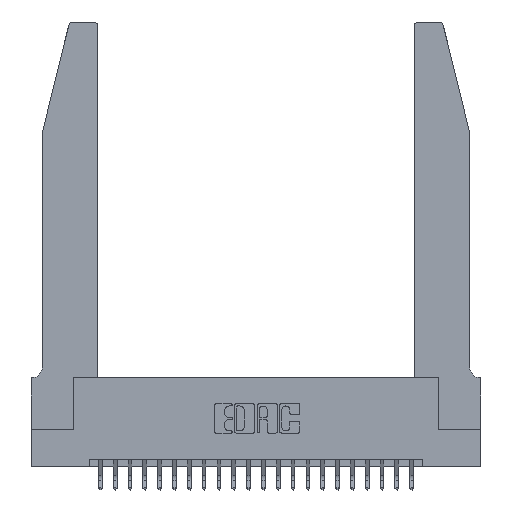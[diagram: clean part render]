
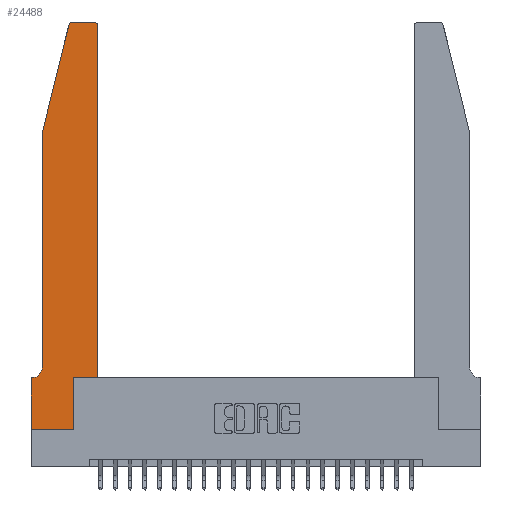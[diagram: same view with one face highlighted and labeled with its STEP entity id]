
A CAD part, top view. The second image highlights one B-rep face of the part: STEP entity #24488.
In plain terms, the highlighted planar face has unit normal (0, 0, 1).
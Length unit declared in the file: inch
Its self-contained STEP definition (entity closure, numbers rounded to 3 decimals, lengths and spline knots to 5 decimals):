
#172 = VERTEX_POINT ( 'NONE', #23364 ) ;
#546 = CARTESIAN_POINT ( 'NONE',  ( 0.2605, 2.75, 0.37 ) ) ;
#727 = CIRCLE ( 'NONE', #18479, 0.07 ) ;
#772 = CARTESIAN_POINT ( 'NONE',  ( 0.0055, 0.42, 0.37 ) ) ;
#1529 = CARTESIAN_POINT ( 'NONE',  ( 0., 0.35, 0.37 ) ) ;
#1618 = VERTEX_POINT ( 'NONE', #3143 ) ;
#1626 = EDGE_CURVE ( 'NONE', #13766, #11503, #6456, .T. ) ;
#1854 = VECTOR ( 'NONE', #22477, 39.37008 ) ;
#2359 = LINE ( 'NONE', #3358, #7561 ) ;
#2394 = EDGE_CURVE ( 'NONE', #13511, #3451, #6112, .T. ) ;
#2552 = DIRECTION ( 'NONE',  ( 0., -1., 0. ) ) ;
#2730 = VECTOR ( 'NONE', #21021, 39.37008 ) ;
#2745 = DIRECTION ( 'NONE',  ( 0., 0., 1. ) ) ;
#2781 = DIRECTION ( 'NONE',  ( -1., 0., 0. ) ) ;
#2784 = CARTESIAN_POINT ( 'NONE',  ( 0.284, 2.75, 0.37 ) ) ;
#2868 = DIRECTION ( 'NONE',  ( 0., 0., 1. ) ) ;
#2999 = VECTOR ( 'NONE', #14228, 39.37008 ) ;
#3043 = CARTESIAN_POINT ( 'NONE',  ( 0.4205, 2.72, 0.37 ) ) ;
#3143 = CARTESIAN_POINT ( 'NONE',  ( 0.0055, 0.35, 0.37 ) ) ;
#3145 = CARTESIAN_POINT ( 'NONE',  ( 0.0755, 2., 0.37 ) ) ;
#3358 = CARTESIAN_POINT ( 'NONE',  ( 0.2865, 0.35, 0.37 ) ) ;
#3451 = VERTEX_POINT ( 'NONE', #13731 ) ;
#3588 = EDGE_CURVE ( 'NONE', #3451, #20982, #6352, .T. ) ;
#3731 = ORIENTED_EDGE ( 'NONE', *, *, #2394, .T. ) ;
#3903 = EDGE_CURVE ( 'NONE', #11503, #10287, #8526, .T. ) ;
#4021 = AXIS2_PLACEMENT_3D ( 'NONE', #3043, #16625, #5015 ) ;
#4498 = CARTESIAN_POINT ( 'NONE',  ( 0., 0., 0.37 ) ) ;
#4783 = VECTOR ( 'NONE', #24114, 39.37008 ) ;
#5015 = DIRECTION ( 'NONE',  ( 1., 0., 0. ) ) ;
#5029 = ORIENTED_EDGE ( 'NONE', *, *, #20060, .T. ) ;
#5086 = EDGE_CURVE ( 'NONE', #10287, #19801, #2359, .T. ) ;
#5288 = CARTESIAN_POINT ( 'NONE',  ( 0.4505, 0.35, 0.37 ) ) ;
#5901 = EDGE_CURVE ( 'NONE', #19801, #16342, #20147, .T. ) ;
#6112 = CIRCLE ( 'NONE', #4021, 0.03 ) ;
#6327 = EDGE_CURVE ( 'NONE', #172, #1618, #727, .T. ) ;
#6352 = LINE ( 'NONE', #546, #2999 ) ;
#6456 = LINE ( 'NONE', #4498, #16154 ) ;
#6720 = CARTESIAN_POINT ( 'NONE',  ( 0.0755, 0.35, 0.37 ) ) ;
#7070 = LINE ( 'NONE', #5288, #1854 ) ;
#7372 = CARTESIAN_POINT ( 'NONE',  ( 0.25487, 2.72718, 0.37 ) ) ;
#7383 = CARTESIAN_POINT ( 'NONE',  ( 0., 0., 0.37 ) ) ;
#7561 = VECTOR ( 'NONE', #11113, 39.37008 ) ;
#7681 = ORIENTED_EDGE ( 'NONE', *, *, #18823, .T. ) ;
#8123 = CARTESIAN_POINT ( 'NONE',  ( 0.4505, 0.35, 0.37 ) ) ;
#8526 = LINE ( 'NONE', #9555, #2730 ) ;
#9133 = AXIS2_PLACEMENT_3D ( 'NONE', #14418, #2745, #16330 ) ;
#9366 = VECTOR ( 'NONE', #20868, 39.37008 ) ;
#9555 = CARTESIAN_POINT ( 'NONE',  ( 0., 0., 0.37 ) ) ;
#9978 = CIRCLE ( 'NONE', #9133, 0.03 ) ;
#10210 = ORIENTED_EDGE ( 'NONE', *, *, #6327, .T. ) ;
#10287 = VERTEX_POINT ( 'NONE', #17101 ) ;
#10933 = EDGE_CURVE ( 'NONE', #19985, #22346, #14527, .T. ) ;
#11113 = DIRECTION ( 'NONE',  ( 0., 1., 0. ) ) ;
#11451 = DIRECTION ( 'NONE',  ( 0., -1., 0. ) ) ;
#11503 = VERTEX_POINT ( 'NONE', #7383 ) ;
#12589 = CARTESIAN_POINT ( 'NONE',  ( 0., 0.35, 0.37 ) ) ;
#12660 = FACE_OUTER_BOUND ( 'NONE', #17041, .T. ) ;
#12776 = CARTESIAN_POINT ( 'NONE',  ( 0.4505, 0.35, 0.37 ) ) ;
#12904 = AXIS2_PLACEMENT_3D ( 'NONE', #12589, #2868, #16449 ) ;
#13511 = VERTEX_POINT ( 'NONE', #23744 ) ;
#13731 = CARTESIAN_POINT ( 'NONE',  ( 0.4205, 2.75, 0.37 ) ) ;
#13766 = VERTEX_POINT ( 'NONE', #1529 ) ;
#14228 = DIRECTION ( 'NONE',  ( -1., 0., 0. ) ) ;
#14418 = CARTESIAN_POINT ( 'NONE',  ( 0.284, 2.72, 0.37 ) ) ;
#14452 = DIRECTION ( 'NONE',  ( 0., 0., -1. ) ) ;
#14527 = LINE ( 'NONE', #17067, #9366 ) ;
#14597 = CARTESIAN_POINT ( 'NONE',  ( 0.2865, 0.35, 0.37 ) ) ;
#16154 = VECTOR ( 'NONE', #2552, 39.37008 ) ;
#16330 = DIRECTION ( 'NONE',  ( 1., 0., 0. ) ) ;
#16342 = VERTEX_POINT ( 'NONE', #8123 ) ;
#16449 = DIRECTION ( 'NONE',  ( 1., 0., 0. ) ) ;
#16625 = DIRECTION ( 'NONE',  ( 0., 0., 1. ) ) ;
#17041 = EDGE_LOOP ( 'NONE', ( #17429, #23014, #19197, #5029, #10210, #20991, #17147, #22149, #18314, #22359, #7681, #3731 ) ) ;
#17067 = CARTESIAN_POINT ( 'NONE',  ( 0.0755, 2., 0.37 ) ) ;
#17101 = CARTESIAN_POINT ( 'NONE',  ( 0.2865, 0., 0.37 ) ) ;
#17147 = ORIENTED_EDGE ( 'NONE', *, *, #1626, .T. ) ;
#17429 = ORIENTED_EDGE ( 'NONE', *, *, #3588, .T. ) ;
#18255 = DIRECTION ( 'NONE',  ( -1., 0., 0. ) ) ;
#18314 = ORIENTED_EDGE ( 'NONE', *, *, #5086, .T. ) ;
#18479 = AXIS2_PLACEMENT_3D ( 'NONE', #772, #14452, #2781 ) ;
#18823 = EDGE_CURVE ( 'NONE', #16342, #13511, #7070, .T. ) ;
#19197 = ORIENTED_EDGE ( 'NONE', *, *, #10933, .T. ) ;
#19501 = LINE ( 'NONE', #6720, #23904 ) ;
#19801 = VERTEX_POINT ( 'NONE', #14597 ) ;
#19985 = VERTEX_POINT ( 'NONE', #7372 ) ;
#20060 = EDGE_CURVE ( 'NONE', #22346, #172, #21993, .T. ) ;
#20147 = LINE ( 'NONE', #12776, #4783 ) ;
#20868 = DIRECTION ( 'NONE',  ( -0.239, -0.971, 0. ) ) ;
#20971 = CARTESIAN_POINT ( 'NONE',  ( 0.0755, 2., 0.37 ) ) ;
#20982 = VERTEX_POINT ( 'NONE', #2784 ) ;
#20991 = ORIENTED_EDGE ( 'NONE', *, *, #22923, .T. ) ;
#21021 = DIRECTION ( 'NONE',  ( 1., 0., 0. ) ) ;
#21425 = VECTOR ( 'NONE', #11451, 39.37008 ) ;
#21993 = LINE ( 'NONE', #20971, #21425 ) ;
#22149 = ORIENTED_EDGE ( 'NONE', *, *, #3903, .T. ) ;
#22346 = VERTEX_POINT ( 'NONE', #3145 ) ;
#22359 = ORIENTED_EDGE ( 'NONE', *, *, #5901, .T. ) ;
#22477 = DIRECTION ( 'NONE',  ( 0., 1., 0. ) ) ;
#22923 = EDGE_CURVE ( 'NONE', #1618, #13766, #19501, .T. ) ;
#23014 = ORIENTED_EDGE ( 'NONE', *, *, #23487, .T. ) ;
#23364 = CARTESIAN_POINT ( 'NONE',  ( 0.0755, 0.42, 0.37 ) ) ;
#23487 = EDGE_CURVE ( 'NONE', #20982, #19985, #9978, .T. ) ;
#23744 = CARTESIAN_POINT ( 'NONE',  ( 0.4505, 2.72, 0.37 ) ) ;
#23904 = VECTOR ( 'NONE', #18255, 39.37008 ) ;
#23938 = PLANE ( 'NONE',  #12904 ) ;
#24114 = DIRECTION ( 'NONE',  ( 1., 0., 0. ) ) ;
#24488 = ADVANCED_FACE ( 'NONE', ( #12660 ), #23938, .T. ) ;
